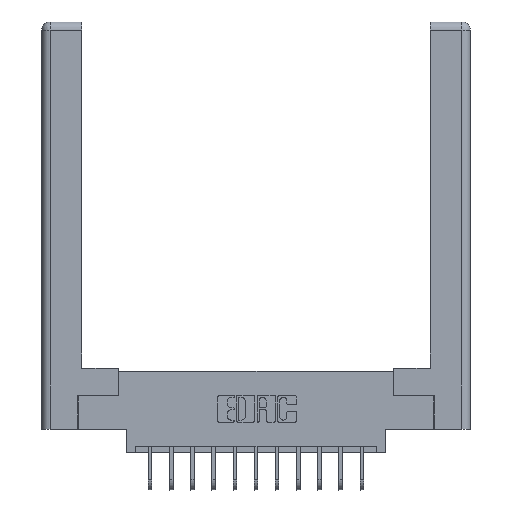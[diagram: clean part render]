
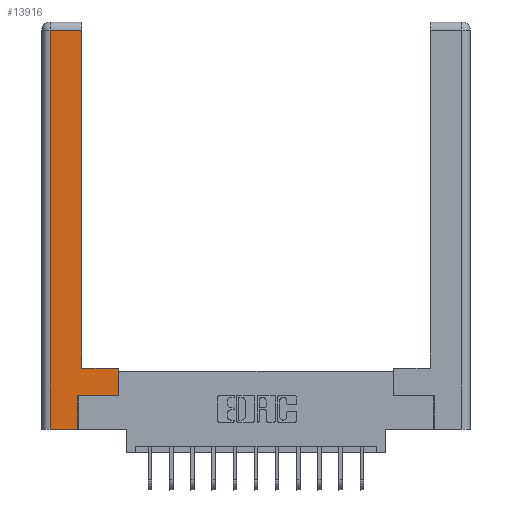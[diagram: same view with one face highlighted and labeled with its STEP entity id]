
A CAD part, top view. The second image highlights one B-rep face of the part: STEP entity #13916.
In plain terms, the highlighted planar face has unit normal (0, 0, 1).
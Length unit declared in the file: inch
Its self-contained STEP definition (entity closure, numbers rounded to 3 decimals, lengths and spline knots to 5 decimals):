
#161 = CARTESIAN_POINT ( 'NONE',  ( 0.265, 0., 0. ) ) ;
#202 = ORIENTED_EDGE ( 'NONE', *, *, #1971, .T. ) ;
#433 = VERTEX_POINT ( 'NONE', #1173 ) ;
#1021 = VERTEX_POINT ( 'NONE', #6357 ) ;
#1173 = CARTESIAN_POINT ( 'NONE',  ( 0.565, 0.45, 0. ) ) ;
#1224 = VERTEX_POINT ( 'NONE', #11797 ) ;
#1396 = EDGE_CURVE ( 'NONE', #12388, #1224, #9058, .T. ) ;
#1730 = DIRECTION ( 'NONE',  ( 1., 0., 0. ) ) ;
#1798 = ORIENTED_EDGE ( 'NONE', *, *, #7307, .T. ) ;
#1879 = DIRECTION ( 'NONE',  ( 0., 1., 0. ) ) ;
#1971 = EDGE_CURVE ( 'NONE', #6465, #10420, #6577, .T. ) ;
#2126 = ORIENTED_EDGE ( 'NONE', *, *, #16295, .T. ) ;
#2195 = DIRECTION ( 'NONE',  ( 0., 1., 0. ) ) ;
#2300 = DIRECTION ( 'NONE',  ( 1., 0., 0. ) ) ;
#2666 = DIRECTION ( 'NONE',  ( 0., 1., 0. ) ) ;
#2670 = LINE ( 'NONE', #15699, #4313 ) ;
#2871 = DIRECTION ( 'NONE',  ( -1., 0., 0. ) ) ;
#3201 = LINE ( 'NONE', #10061, #12065 ) ;
#3299 = DIRECTION ( 'NONE',  ( -1., 0., 0. ) ) ;
#3369 = CARTESIAN_POINT ( 'NONE',  ( 0.265, 0.245, 0. ) ) ;
#4065 = CARTESIAN_POINT ( 'NONE',  ( 0.0615, 2.94, 0. ) ) ;
#4266 = EDGE_CURVE ( 'NONE', #1021, #12388, #2670, .T. ) ;
#4283 = ORIENTED_EDGE ( 'NONE', *, *, #1396, .T. ) ;
#4313 = VECTOR ( 'NONE', #2300, 39.37008 ) ;
#4908 = ORIENTED_EDGE ( 'NONE', *, *, #7089, .T. ) ;
#6002 = DIRECTION ( 'NONE',  ( 0., -1., 0. ) ) ;
#6231 = CARTESIAN_POINT ( 'NONE',  ( 0., 0., 0. ) ) ;
#6357 = CARTESIAN_POINT ( 'NONE',  ( 0.0615, 0., 0. ) ) ;
#6465 = VERTEX_POINT ( 'NONE', #8366 ) ;
#6565 = FACE_OUTER_BOUND ( 'NONE', #16212, .T. ) ;
#6577 = LINE ( 'NONE', #13231, #13617 ) ;
#6673 = CARTESIAN_POINT ( 'NONE',  ( 0.295, 2.94, 0. ) ) ;
#6676 = LINE ( 'NONE', #16349, #12884 ) ;
#7089 = EDGE_CURVE ( 'NONE', #1224, #13926, #6676, .T. ) ;
#7307 = EDGE_CURVE ( 'NONE', #433, #6465, #3201, .T. ) ;
#7711 = VERTEX_POINT ( 'NONE', #12159 ) ;
#8209 = VECTOR ( 'NONE', #2195, 39.37008 ) ;
#8366 = CARTESIAN_POINT ( 'NONE',  ( 0.295, 0.45, 0. ) ) ;
#8386 = EDGE_CURVE ( 'NONE', #13926, #433, #16388, .T. ) ;
#8435 = CARTESIAN_POINT ( 'NONE',  ( 0.565, 0.45, 0. ) ) ;
#9058 = LINE ( 'NONE', #3369, #8209 ) ;
#9711 = LINE ( 'NONE', #4065, #12643 ) ;
#10061 = CARTESIAN_POINT ( 'NONE',  ( 0.295, 0.45, 0. ) ) ;
#10420 = VERTEX_POINT ( 'NONE', #6673 ) ;
#10989 = EDGE_CURVE ( 'NONE', #10420, #7711, #9711, .T. ) ;
#11600 = CARTESIAN_POINT ( 'NONE',  ( 0.565, 0.245, 0. ) ) ;
#11699 = AXIS2_PLACEMENT_3D ( 'NONE', #6231, #14294, #16989 ) ;
#11797 = CARTESIAN_POINT ( 'NONE',  ( 0.265, 0.245, 0. ) ) ;
#12065 = VECTOR ( 'NONE', #3299, 39.37008 ) ;
#12159 = CARTESIAN_POINT ( 'NONE',  ( 0.0615, 2.94, 0. ) ) ;
#12388 = VERTEX_POINT ( 'NONE', #161 ) ;
#12643 = VECTOR ( 'NONE', #2871, 39.37008 ) ;
#12883 = PLANE ( 'NONE',  #11699 ) ;
#12884 = VECTOR ( 'NONE', #1730, 39.37008 ) ;
#13231 = CARTESIAN_POINT ( 'NONE',  ( 0.295, 3., 0. ) ) ;
#13335 = ORIENTED_EDGE ( 'NONE', *, *, #10989, .T. ) ;
#13617 = VECTOR ( 'NONE', #2666, 39.37008 ) ;
#13916 = ADVANCED_FACE ( 'NONE', ( #6565 ), #12883, .F. ) ;
#13923 = CARTESIAN_POINT ( 'NONE',  ( 0.0615, 0., 0. ) ) ;
#13926 = VERTEX_POINT ( 'NONE', #11600 ) ;
#14294 = DIRECTION ( 'NONE',  ( 0., 0., -1. ) ) ;
#15445 = VECTOR ( 'NONE', #6002, 39.37008 ) ;
#15560 = ORIENTED_EDGE ( 'NONE', *, *, #4266, .T. ) ;
#15620 = ORIENTED_EDGE ( 'NONE', *, *, #8386, .T. ) ;
#15699 = CARTESIAN_POINT ( 'NONE',  ( 0.265, 0., 0. ) ) ;
#15876 = LINE ( 'NONE', #13923, #15445 ) ;
#16212 = EDGE_LOOP ( 'NONE', ( #202, #13335, #2126, #15560, #4283, #4908, #15620, #1798 ) ) ;
#16295 = EDGE_CURVE ( 'NONE', #7711, #1021, #15876, .T. ) ;
#16349 = CARTESIAN_POINT ( 'NONE',  ( 0.565, 0.245, 0. ) ) ;
#16388 = LINE ( 'NONE', #8435, #17001 ) ;
#16989 = DIRECTION ( 'NONE',  ( -1., 0., 0. ) ) ;
#17001 = VECTOR ( 'NONE', #1879, 39.37008 ) ;
